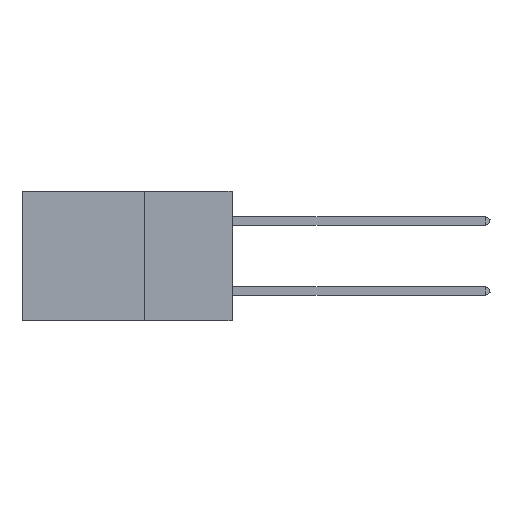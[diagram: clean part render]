
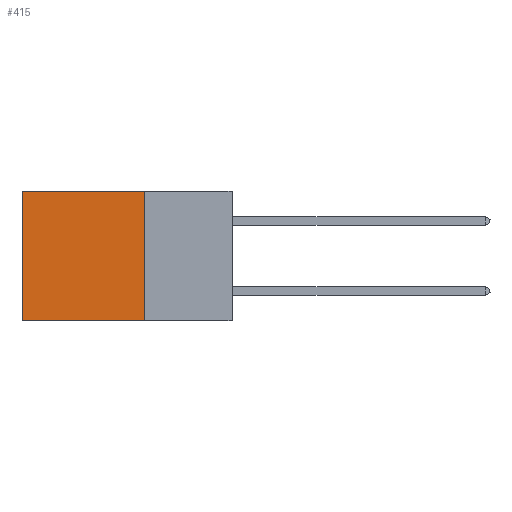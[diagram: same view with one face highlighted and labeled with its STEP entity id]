
A CAD part, left-side view. The second image highlights one B-rep face of the part: STEP entity #415.
In plain terms, the highlighted planar face has unit normal (-1, 0, 0).
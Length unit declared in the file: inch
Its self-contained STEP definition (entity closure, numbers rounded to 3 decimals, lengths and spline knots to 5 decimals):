
#415 = ADVANCED_FACE ( 'NONE', ( #38834 ), #11994, .F. ) ;
#1625 = CARTESIAN_POINT ( 'NONE',  ( 0.2875, 0.25, -0.37 ) ) ;
#2953 = ORIENTED_EDGE ( 'NONE', *, *, #17000, .F. ) ;
#4276 = VECTOR ( 'NONE', #31019, 39.37008 ) ;
#5864 = CARTESIAN_POINT ( 'NONE',  ( 0.2875, 0.6, 0. ) ) ;
#7255 = EDGE_LOOP ( 'NONE', ( #33442, #23004, #2953, #29861 ) ) ;
#7426 = CARTESIAN_POINT ( 'NONE',  ( 0.2875, 0.25, 0. ) ) ;
#11701 = DIRECTION ( 'NONE',  ( 0., 1., 0. ) ) ;
#11994 = PLANE ( 'NONE',  #45635 ) ;
#15537 = DIRECTION ( 'NONE',  ( 0., 0., -1. ) ) ;
#15869 = EDGE_CURVE ( 'NONE', #45762, #42108, #37056, .T. ) ;
#16312 = EDGE_CURVE ( 'NONE', #43056, #20371, #46551, .T. ) ;
#17000 = EDGE_CURVE ( 'NONE', #45762, #43056, #29659, .T. ) ;
#17210 = CARTESIAN_POINT ( 'NONE',  ( 0.2875, 0.25, 0. ) ) ;
#20081 = VECTOR ( 'NONE', #15537, 39.37008 ) ;
#20371 = VERTEX_POINT ( 'NONE', #40613 ) ;
#21891 = CARTESIAN_POINT ( 'NONE',  ( 0.2875, 0.25, -0.37 ) ) ;
#22777 = CARTESIAN_POINT ( 'NONE',  ( 0.2875, 0.25, 0. ) ) ;
#23004 = ORIENTED_EDGE ( 'NONE', *, *, #16312, .F. ) ;
#26131 = DIRECTION ( 'NONE',  ( 0., 0., -1. ) ) ;
#26582 = CARTESIAN_POINT ( 'NONE',  ( 0.2875, 0.25, 0. ) ) ;
#27490 = VECTOR ( 'NONE', #35268, 39.37008 ) ;
#29659 = LINE ( 'NONE', #22777, #20081 ) ;
#29861 = ORIENTED_EDGE ( 'NONE', *, *, #15869, .T. ) ;
#30201 = DIRECTION ( 'NONE',  ( 1., 0., 0. ) ) ;
#31019 = DIRECTION ( 'NONE',  ( 0., 0., -1. ) ) ;
#32535 = VECTOR ( 'NONE', #11701, 39.37008 ) ;
#33442 = ORIENTED_EDGE ( 'NONE', *, *, #37675, .T. ) ;
#35268 = DIRECTION ( 'NONE',  ( 0., 1., 0. ) ) ;
#37056 = LINE ( 'NONE', #17210, #27490 ) ;
#37675 = EDGE_CURVE ( 'NONE', #42108, #20371, #38618, .T. ) ;
#38618 = LINE ( 'NONE', #5864, #4276 ) ;
#38834 = FACE_OUTER_BOUND ( 'NONE', #7255, .T. ) ;
#40107 = CARTESIAN_POINT ( 'NONE',  ( 0.2875, 0.6, 0. ) ) ;
#40613 = CARTESIAN_POINT ( 'NONE',  ( 0.2875, 0.6, -0.37 ) ) ;
#42108 = VERTEX_POINT ( 'NONE', #40107 ) ;
#43056 = VERTEX_POINT ( 'NONE', #1625 ) ;
#45635 = AXIS2_PLACEMENT_3D ( 'NONE', #26582, #30201, #26131 ) ;
#45762 = VERTEX_POINT ( 'NONE', #7426 ) ;
#46551 = LINE ( 'NONE', #21891, #32535 ) ;
